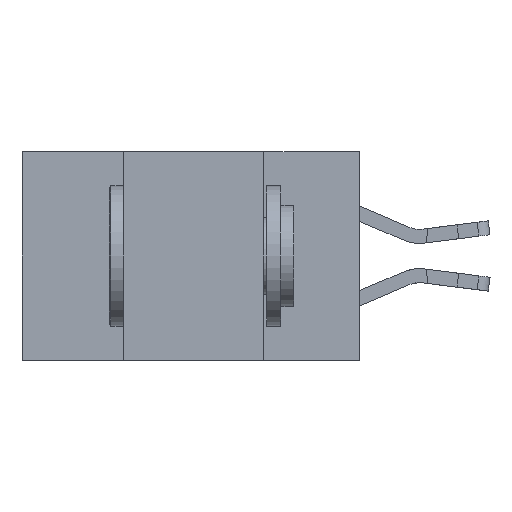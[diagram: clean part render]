
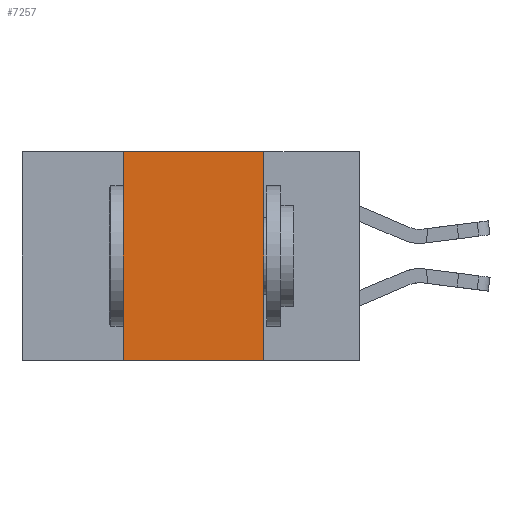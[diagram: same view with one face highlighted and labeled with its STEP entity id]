
A CAD part, left-side view. The second image highlights one B-rep face of the part: STEP entity #7257.
In plain terms, the highlighted planar face has unit normal (-1, 0, 0).
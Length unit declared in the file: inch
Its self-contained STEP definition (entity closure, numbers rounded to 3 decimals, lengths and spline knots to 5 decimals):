
#116 = VERTEX_POINT ( 'NONE', #3314 ) ;
#237 = VERTEX_POINT ( 'NONE', #14152 ) ;
#716 = LINE ( 'NONE', #13757, #19080 ) ;
#1673 = VECTOR ( 'NONE', #5931, 39.37008 ) ;
#2863 = CARTESIAN_POINT ( 'NONE',  ( 0., 0.42, 0. ) ) ;
#3314 = CARTESIAN_POINT ( 'NONE',  ( 0., 0.17, 0. ) ) ;
#4319 = VERTEX_POINT ( 'NONE', #10565 ) ;
#5904 = EDGE_CURVE ( 'NONE', #237, #4319, #716, .T. ) ;
#5931 = DIRECTION ( 'NONE',  ( 0., -1., 0. ) ) ;
#6186 = ORIENTED_EDGE ( 'NONE', *, *, #21738, .F. ) ;
#6542 = LINE ( 'NONE', #18238, #1673 ) ;
#6762 = DIRECTION ( 'NONE',  ( 0., -1., 0. ) ) ;
#6928 = ORIENTED_EDGE ( 'NONE', *, *, #11720, .F. ) ;
#7257 = ADVANCED_FACE ( 'NONE', ( #20083 ), #12283, .F. ) ;
#7586 = ORIENTED_EDGE ( 'NONE', *, *, #16863, .F. ) ;
#8084 = ORIENTED_EDGE ( 'NONE', *, *, #5904, .T. ) ;
#8318 = DIRECTION ( 'NONE',  ( 0., 0., 1. ) ) ;
#8664 = CARTESIAN_POINT ( 'NONE',  ( 0., 0.17, 0. ) ) ;
#8781 = DIRECTION ( 'NONE',  ( 1., 0., 0. ) ) ;
#10565 = CARTESIAN_POINT ( 'NONE',  ( 0., 0.17, -0.37 ) ) ;
#11720 = EDGE_CURVE ( 'NONE', #12782, #116, #6542, .T. ) ;
#12151 = VECTOR ( 'NONE', #22585, 39.37008 ) ;
#12229 = EDGE_LOOP ( 'NONE', ( #6186, #6928, #7586, #8084 ) ) ;
#12283 = PLANE ( 'NONE',  #14323 ) ;
#12420 = VECTOR ( 'NONE', #8318, 39.37008 ) ;
#12782 = VERTEX_POINT ( 'NONE', #16404 ) ;
#13757 = CARTESIAN_POINT ( 'NONE',  ( 0., 0.6, -0.37 ) ) ;
#14152 = CARTESIAN_POINT ( 'NONE',  ( 0., 0.42, -0.37 ) ) ;
#14323 = AXIS2_PLACEMENT_3D ( 'NONE', #19270, #8781, #20989 ) ;
#16404 = CARTESIAN_POINT ( 'NONE',  ( 0., 0.42, 0. ) ) ;
#16863 = EDGE_CURVE ( 'NONE', #237, #12782, #17600, .T. ) ;
#17600 = LINE ( 'NONE', #2863, #12420 ) ;
#18238 = CARTESIAN_POINT ( 'NONE',  ( 0., 0.6, 0. ) ) ;
#19080 = VECTOR ( 'NONE', #6762, 39.37008 ) ;
#19270 = CARTESIAN_POINT ( 'NONE',  ( 0., 0.6, 0. ) ) ;
#20083 = FACE_OUTER_BOUND ( 'NONE', #12229, .T. ) ;
#20827 = LINE ( 'NONE', #8664, #12151 ) ;
#20989 = DIRECTION ( 'NONE',  ( 0., 0., -1. ) ) ;
#21738 = EDGE_CURVE ( 'NONE', #116, #4319, #20827, .T. ) ;
#22585 = DIRECTION ( 'NONE',  ( 0., 0., -1. ) ) ;
